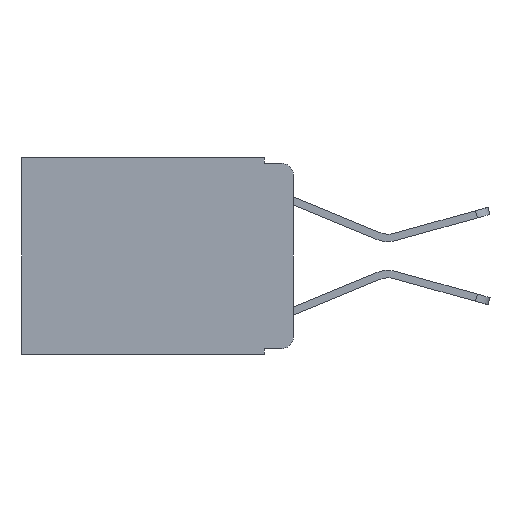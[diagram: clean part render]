
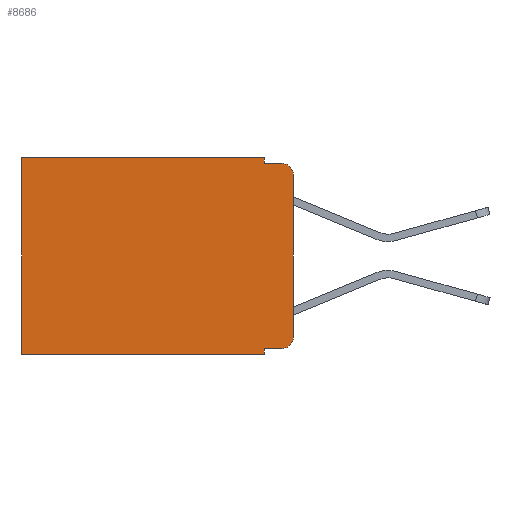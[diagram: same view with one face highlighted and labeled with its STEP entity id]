
A CAD part, left-side view. The second image highlights one B-rep face of the part: STEP entity #8686.
In plain terms, the highlighted planar face has unit normal (-1, 0, 0).
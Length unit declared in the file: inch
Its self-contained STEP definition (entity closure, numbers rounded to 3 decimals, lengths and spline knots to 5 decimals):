
#59 = VECTOR ( 'NONE', #12566, 39.37008 ) ;
#204 = CIRCLE ( 'NONE', #3383, 0.02 ) ;
#353 = CARTESIAN_POINT ( 'NONE',  ( 0.298, 0.02, -0.313 ) ) ;
#423 = VECTOR ( 'NONE', #8559, 39.37008 ) ;
#506 = CARTESIAN_POINT ( 'NONE',  ( 0.298, 0.473, 0. ) ) ;
#717 = CARTESIAN_POINT ( 'NONE',  ( 0.298, 0., -0.343 ) ) ;
#997 = DIRECTION ( 'NONE',  ( -1., 0., 0. ) ) ;
#1047 = CARTESIAN_POINT ( 'NONE',  ( 0.298, 0.051, -0.333 ) ) ;
#1056 = ORIENTED_EDGE ( 'NONE', *, *, #13034, .T. ) ;
#1080 = VECTOR ( 'NONE', #5531, 39.37008 ) ;
#1310 = CARTESIAN_POINT ( 'NONE',  ( 0.298, 0., 0. ) ) ;
#1511 = VECTOR ( 'NONE', #10936, 39.37008 ) ;
#2065 = VERTEX_POINT ( 'NONE', #15545 ) ;
#2782 = CARTESIAN_POINT ( 'NONE',  ( 0.298, 0.02, -0.01 ) ) ;
#3383 = AXIS2_PLACEMENT_3D ( 'NONE', #15310, #997, #4451 ) ;
#3512 = EDGE_LOOP ( 'NONE', ( #14139, #9736, #7543, #6797, #1056, #11634, #13358, #11030, #14641, #4599 ) ) ;
#3892 = DIRECTION ( 'NONE',  ( 0., 0., -1. ) ) ;
#4092 = DIRECTION ( 'NONE',  ( 0., 0., -1. ) ) ;
#4144 = CARTESIAN_POINT ( 'NONE',  ( 0.298, 0.051, 0. ) ) ;
#4202 = CARTESIAN_POINT ( 'NONE',  ( 0.298, 0., -0.313 ) ) ;
#4254 = VERTEX_POINT ( 'NONE', #11922 ) ;
#4451 = DIRECTION ( 'NONE',  ( 0., 0., -1. ) ) ;
#4599 = ORIENTED_EDGE ( 'NONE', *, *, #10986, .T. ) ;
#4638 = LINE ( 'NONE', #717, #59 ) ;
#4767 = DIRECTION ( 'NONE',  ( 1., 0., 0. ) ) ;
#4979 = VERTEX_POINT ( 'NONE', #14328 ) ;
#5058 = CARTESIAN_POINT ( 'NONE',  ( 0.298, 0.051, 0. ) ) ;
#5109 = EDGE_CURVE ( 'NONE', #10815, #14582, #12493, .T. ) ;
#5443 = VECTOR ( 'NONE', #13745, 39.37008 ) ;
#5531 = DIRECTION ( 'NONE',  ( 0., 0., -1. ) ) ;
#5690 = CARTESIAN_POINT ( 'NONE',  ( 0.298, 0.473, -0.343 ) ) ;
#6434 = CARTESIAN_POINT ( 'NONE',  ( 0.298, 0.02, -0.333 ) ) ;
#6454 = DIRECTION ( 'NONE',  ( 0., 0., -1. ) ) ;
#6797 = ORIENTED_EDGE ( 'NONE', *, *, #13963, .F. ) ;
#6887 = VERTEX_POINT ( 'NONE', #10752 ) ;
#6934 = FACE_OUTER_BOUND ( 'NONE', #3512, .T. ) ;
#7118 = LINE ( 'NONE', #4144, #8664 ) ;
#7543 = ORIENTED_EDGE ( 'NONE', *, *, #5109, .F. ) ;
#7708 = EDGE_CURVE ( 'NONE', #13993, #14816, #8116, .T. ) ;
#7836 = CARTESIAN_POINT ( 'NONE',  ( 0.298, 0., 0. ) ) ;
#7932 = VECTOR ( 'NONE', #3892, 39.37008 ) ;
#8116 = LINE ( 'NONE', #1310, #7932 ) ;
#8534 = EDGE_CURVE ( 'NONE', #2065, #11103, #4638, .T. ) ;
#8559 = DIRECTION ( 'NONE',  ( 0., 0., -1. ) ) ;
#8664 = VECTOR ( 'NONE', #4092, 39.37008 ) ;
#8686 = ADVANCED_FACE ( 'NONE', ( #6934 ), #11956, .F. ) ;
#8734 = VECTOR ( 'NONE', #13049, 39.37008 ) ;
#8971 = DIRECTION ( 'NONE',  ( -1., 0., 0. ) ) ;
#9736 = ORIENTED_EDGE ( 'NONE', *, *, #14439, .T. ) ;
#9752 = AXIS2_PLACEMENT_3D ( 'NONE', #15625, #4767, #12012 ) ;
#10056 = EDGE_CURVE ( 'NONE', #4254, #2065, #7118, .T. ) ;
#10136 = LINE ( 'NONE', #5058, #423 ) ;
#10752 = CARTESIAN_POINT ( 'NONE',  ( 0.298, 0.473, 0. ) ) ;
#10792 = LINE ( 'NONE', #506, #1080 ) ;
#10815 = VERTEX_POINT ( 'NONE', #12263 ) ;
#10883 = CARTESIAN_POINT ( 'NONE',  ( 0.298, 0.051, -0.01 ) ) ;
#10936 = DIRECTION ( 'NONE',  ( 0., -1., 0. ) ) ;
#10960 = VERTEX_POINT ( 'NONE', #6434 ) ;
#10986 = EDGE_CURVE ( 'NONE', #10960, #14816, #11595, .T. ) ;
#11030 = ORIENTED_EDGE ( 'NONE', *, *, #10056, .F. ) ;
#11103 = VERTEX_POINT ( 'NONE', #5690 ) ;
#11287 = AXIS2_PLACEMENT_3D ( 'NONE', #353, #8971, #6454 ) ;
#11595 = CIRCLE ( 'NONE', #11287, 0.02 ) ;
#11634 = ORIENTED_EDGE ( 'NONE', *, *, #12209, .T. ) ;
#11874 = LINE ( 'NONE', #7836, #5443 ) ;
#11922 = CARTESIAN_POINT ( 'NONE',  ( 0.298, 0.051, -0.333 ) ) ;
#11956 = PLANE ( 'NONE',  #9752 ) ;
#12012 = DIRECTION ( 'NONE',  ( 0., 0., -1. ) ) ;
#12109 = EDGE_CURVE ( 'NONE', #4254, #10960, #12428, .T. ) ;
#12209 = EDGE_CURVE ( 'NONE', #6887, #11103, #10792, .T. ) ;
#12263 = CARTESIAN_POINT ( 'NONE',  ( 0.298, 0.051, -0.01 ) ) ;
#12428 = LINE ( 'NONE', #1047, #8734 ) ;
#12493 = LINE ( 'NONE', #10883, #1511 ) ;
#12566 = DIRECTION ( 'NONE',  ( 0., 1., 0. ) ) ;
#13034 = EDGE_CURVE ( 'NONE', #4979, #6887, #11874, .T. ) ;
#13049 = DIRECTION ( 'NONE',  ( 0., -1., 0. ) ) ;
#13358 = ORIENTED_EDGE ( 'NONE', *, *, #8534, .F. ) ;
#13382 = CARTESIAN_POINT ( 'NONE',  ( 0.298, 0., -0.03 ) ) ;
#13745 = DIRECTION ( 'NONE',  ( 0., 1., 0. ) ) ;
#13963 = EDGE_CURVE ( 'NONE', #4979, #10815, #10136, .T. ) ;
#13993 = VERTEX_POINT ( 'NONE', #13382 ) ;
#14139 = ORIENTED_EDGE ( 'NONE', *, *, #7708, .F. ) ;
#14328 = CARTESIAN_POINT ( 'NONE',  ( 0.298, 0.051, 0. ) ) ;
#14439 = EDGE_CURVE ( 'NONE', #13993, #14582, #204, .T. ) ;
#14582 = VERTEX_POINT ( 'NONE', #2782 ) ;
#14641 = ORIENTED_EDGE ( 'NONE', *, *, #12109, .T. ) ;
#14816 = VERTEX_POINT ( 'NONE', #4202 ) ;
#15310 = CARTESIAN_POINT ( 'NONE',  ( 0.298, 0.02, -0.03 ) ) ;
#15545 = CARTESIAN_POINT ( 'NONE',  ( 0.298, 0.051, -0.343 ) ) ;
#15625 = CARTESIAN_POINT ( 'NONE',  ( 0.298, 0., 0. ) ) ;
